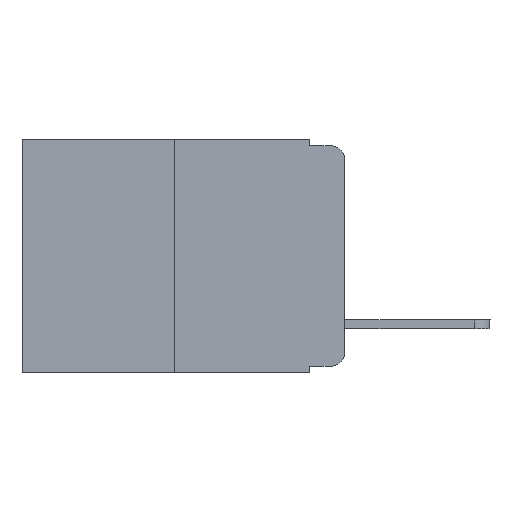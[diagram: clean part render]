
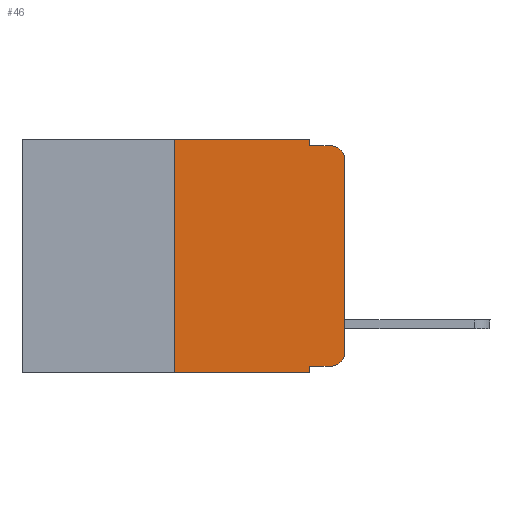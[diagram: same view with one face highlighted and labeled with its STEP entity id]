
A CAD part, left-side view. The second image highlights one B-rep face of the part: STEP entity #46.
In plain terms, the highlighted planar face has unit normal (-1, 0, 0).
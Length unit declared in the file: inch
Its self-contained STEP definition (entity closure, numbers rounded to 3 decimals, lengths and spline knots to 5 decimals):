
#14 = VECTOR ( 'NONE', #6966, 39.37008 ) ;
#46 = ADVANCED_FACE ( 'NONE', ( #4939 ), #713, .F. ) ;
#422 = VECTOR ( 'NONE', #2599, 39.37008 ) ;
#462 = EDGE_CURVE ( 'NONE', #2325, #7365, #11428, .T. ) ;
#544 = DIRECTION ( 'NONE',  ( 0., -1., 0. ) ) ;
#713 = PLANE ( 'NONE',  #8978 ) ;
#718 = CARTESIAN_POINT ( 'NONE',  ( 0., 0.051, -0.343 ) ) ;
#995 = VERTEX_POINT ( 'NONE', #11331 ) ;
#1119 = CARTESIAN_POINT ( 'NONE',  ( 0., 0.051, 0. ) ) ;
#1202 = DIRECTION ( 'NONE',  ( -1., 0., 0. ) ) ;
#1294 = EDGE_CURVE ( 'NONE', #11090, #10193, #6574, .T. ) ;
#1511 = VERTEX_POINT ( 'NONE', #2242 ) ;
#1643 = EDGE_CURVE ( 'NONE', #2325, #6590, #12799, .T. ) ;
#1924 = VECTOR ( 'NONE', #2024, 39.37008 ) ;
#2024 = DIRECTION ( 'NONE',  ( 0., 0., -1. ) ) ;
#2242 = CARTESIAN_POINT ( 'NONE',  ( 0., 0.25, -0.343 ) ) ;
#2299 = EDGE_CURVE ( 'NONE', #3615, #995, #6257, .T. ) ;
#2325 = VERTEX_POINT ( 'NONE', #9428 ) ;
#2360 = CARTESIAN_POINT ( 'NONE',  ( 0., 0.473, 0. ) ) ;
#2365 = ORIENTED_EDGE ( 'NONE', *, *, #3241, .F. ) ;
#2454 = LINE ( 'NONE', #12418, #422 ) ;
#2599 = DIRECTION ( 'NONE',  ( 0., 0., 1. ) ) ;
#3142 = ORIENTED_EDGE ( 'NONE', *, *, #2299, .T. ) ;
#3170 = LINE ( 'NONE', #2360, #10035 ) ;
#3241 = EDGE_CURVE ( 'NONE', #1511, #12041, #2454, .T. ) ;
#3615 = VERTEX_POINT ( 'NONE', #12206 ) ;
#3824 = DIRECTION ( 'NONE',  ( 0., 0., 1. ) ) ;
#4115 = CARTESIAN_POINT ( 'NONE',  ( 0., 0.02, -0.03 ) ) ;
#4360 = EDGE_LOOP ( 'NONE', ( #3142, #7504, #10744, #5656, #5805, #2365, #10285, #8441, #5818, #12536 ) ) ;
#4364 = EDGE_CURVE ( 'NONE', #10193, #9489, #9747, .T. ) ;
#4844 = CARTESIAN_POINT ( 'NONE',  ( 0., 0.473, 0. ) ) ;
#4939 = FACE_OUTER_BOUND ( 'NONE', #4360, .T. ) ;
#5059 = LINE ( 'NONE', #7550, #7068 ) ;
#5656 = ORIENTED_EDGE ( 'NONE', *, *, #1294, .F. ) ;
#5744 = EDGE_CURVE ( 'NONE', #12041, #11090, #3170, .T. ) ;
#5805 = ORIENTED_EDGE ( 'NONE', *, *, #5744, .F. ) ;
#5817 = VECTOR ( 'NONE', #8564, 39.37008 ) ;
#5818 = ORIENTED_EDGE ( 'NONE', *, *, #1643, .T. ) ;
#5877 = EDGE_CURVE ( 'NONE', #1511, #7365, #5059, .T. ) ;
#6084 = CIRCLE ( 'NONE', #7799, 0.02 ) ;
#6127 = DIRECTION ( 'NONE',  ( 0., 0., -1. ) ) ;
#6153 = CARTESIAN_POINT ( 'NONE',  ( 0., 0.051, -0.01 ) ) ;
#6257 = LINE ( 'NONE', #9469, #11220 ) ;
#6574 = LINE ( 'NONE', #1119, #14 ) ;
#6590 = VERTEX_POINT ( 'NONE', #12403 ) ;
#6623 = CARTESIAN_POINT ( 'NONE',  ( 0., 0.051, -0.01 ) ) ;
#6966 = DIRECTION ( 'NONE',  ( 0., 0., -1. ) ) ;
#7068 = VECTOR ( 'NONE', #9349, 39.37008 ) ;
#7365 = VERTEX_POINT ( 'NONE', #718 ) ;
#7428 = DIRECTION ( 'NONE',  ( -1., 0., 0. ) ) ;
#7504 = ORIENTED_EDGE ( 'NONE', *, *, #9732, .T. ) ;
#7550 = CARTESIAN_POINT ( 'NONE',  ( 0., 0.473, -0.343 ) ) ;
#7742 = DIRECTION ( 'NONE',  ( 0., 0., -1. ) ) ;
#7799 = AXIS2_PLACEMENT_3D ( 'NONE', #11383, #7428, #11422 ) ;
#8003 = EDGE_CURVE ( 'NONE', #6590, #3615, #6084, .T. ) ;
#8145 = AXIS2_PLACEMENT_3D ( 'NONE', #4115, #1202, #6127 ) ;
#8441 = ORIENTED_EDGE ( 'NONE', *, *, #462, .F. ) ;
#8564 = DIRECTION ( 'NONE',  ( 0., -1., 0. ) ) ;
#8813 = CARTESIAN_POINT ( 'NONE',  ( 0., 0.02, -0.01 ) ) ;
#8831 = DIRECTION ( 'NONE',  ( 1., 0., 0. ) ) ;
#8978 = AXIS2_PLACEMENT_3D ( 'NONE', #4844, #8831, #7742 ) ;
#9349 = DIRECTION ( 'NONE',  ( 0., -1., 0. ) ) ;
#9428 = CARTESIAN_POINT ( 'NONE',  ( 0., 0.051, -0.333 ) ) ;
#9469 = CARTESIAN_POINT ( 'NONE',  ( 0., 0., 0. ) ) ;
#9489 = VERTEX_POINT ( 'NONE', #8813 ) ;
#9732 = EDGE_CURVE ( 'NONE', #995, #9489, #12714, .T. ) ;
#9747 = LINE ( 'NONE', #6623, #9892 ) ;
#9892 = VECTOR ( 'NONE', #544, 39.37008 ) ;
#10035 = VECTOR ( 'NONE', #10428, 39.37008 ) ;
#10102 = CARTESIAN_POINT ( 'NONE',  ( 0., 0.25, 0. ) ) ;
#10193 = VERTEX_POINT ( 'NONE', #6153 ) ;
#10285 = ORIENTED_EDGE ( 'NONE', *, *, #5877, .T. ) ;
#10428 = DIRECTION ( 'NONE',  ( 0., -1., 0. ) ) ;
#10642 = CARTESIAN_POINT ( 'NONE',  ( 0., 0.051, 0. ) ) ;
#10744 = ORIENTED_EDGE ( 'NONE', *, *, #4364, .F. ) ;
#11090 = VERTEX_POINT ( 'NONE', #10642 ) ;
#11220 = VECTOR ( 'NONE', #3824, 39.37008 ) ;
#11331 = CARTESIAN_POINT ( 'NONE',  ( 0., 0., -0.03 ) ) ;
#11383 = CARTESIAN_POINT ( 'NONE',  ( 0., 0.02, -0.313 ) ) ;
#11389 = CARTESIAN_POINT ( 'NONE',  ( 0., 0.051, -0.333 ) ) ;
#11422 = DIRECTION ( 'NONE',  ( 0., 0., -1. ) ) ;
#11428 = LINE ( 'NONE', #12915, #1924 ) ;
#12041 = VERTEX_POINT ( 'NONE', #10102 ) ;
#12206 = CARTESIAN_POINT ( 'NONE',  ( 0., 0., -0.313 ) ) ;
#12403 = CARTESIAN_POINT ( 'NONE',  ( 0., 0.02, -0.333 ) ) ;
#12418 = CARTESIAN_POINT ( 'NONE',  ( 0., 0.25, 0. ) ) ;
#12536 = ORIENTED_EDGE ( 'NONE', *, *, #8003, .T. ) ;
#12714 = CIRCLE ( 'NONE', #8145, 0.02 ) ;
#12799 = LINE ( 'NONE', #11389, #5817 ) ;
#12915 = CARTESIAN_POINT ( 'NONE',  ( 0., 0.051, 0. ) ) ;
